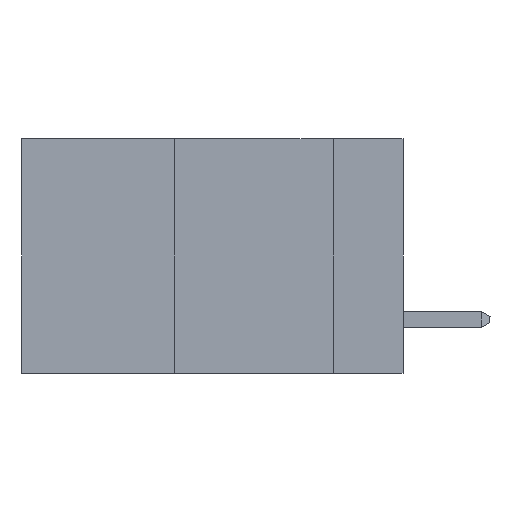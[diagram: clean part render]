
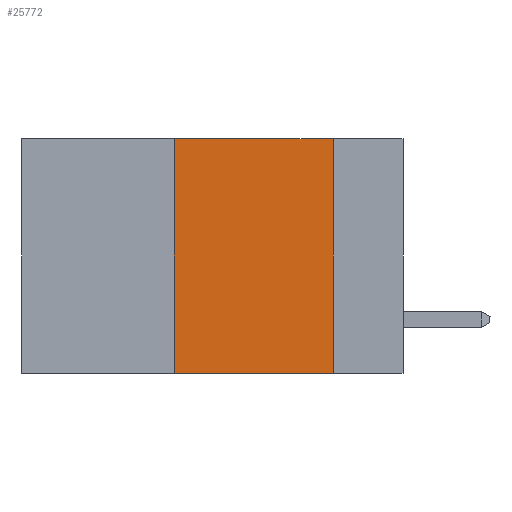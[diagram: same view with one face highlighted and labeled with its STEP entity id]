
A CAD part, left-side view. The second image highlights one B-rep face of the part: STEP entity #25772.
In plain terms, the highlighted planar face has unit normal (-1, 0, 0).
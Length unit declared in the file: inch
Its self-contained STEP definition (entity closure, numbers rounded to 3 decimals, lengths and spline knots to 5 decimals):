
#14 = VECTOR ( 'NONE', #22375, 39.37008 ) ;
#524 = EDGE_LOOP ( 'NONE', ( #15929, #22071, #20313, #9872 ) ) ;
#2654 = DIRECTION ( 'NONE',  ( 0., 0., 1. ) ) ;
#3019 = EDGE_CURVE ( 'NONE', #25509, #14269, #8881, .T. ) ;
#3433 = LINE ( 'NONE', #7960, #14 ) ;
#7960 = CARTESIAN_POINT ( 'NONE',  ( 0., 0.6, 0. ) ) ;
#8402 = CARTESIAN_POINT ( 'NONE',  ( 0., 0.11, 0. ) ) ;
#8881 = LINE ( 'NONE', #13435, #9071 ) ;
#9071 = VECTOR ( 'NONE', #18266, 39.37008 ) ;
#9872 = ORIENTED_EDGE ( 'NONE', *, *, #3019, .T. ) ;
#10600 = CARTESIAN_POINT ( 'NONE',  ( 0., 0.11, 0. ) ) ;
#10876 = CARTESIAN_POINT ( 'NONE',  ( 0., 0.11, -0.37 ) ) ;
#12364 = CARTESIAN_POINT ( 'NONE',  ( 0., 0.36, -0.37 ) ) ;
#13435 = CARTESIAN_POINT ( 'NONE',  ( 0., 0.6, -0.37 ) ) ;
#13705 = VERTEX_POINT ( 'NONE', #10600 ) ;
#13859 = AXIS2_PLACEMENT_3D ( 'NONE', #21410, #26269, #28163 ) ;
#14269 = VERTEX_POINT ( 'NONE', #10876 ) ;
#14543 = CARTESIAN_POINT ( 'NONE',  ( 0., 0.36, 0. ) ) ;
#15761 = LINE ( 'NONE', #8402, #27824 ) ;
#15929 = ORIENTED_EDGE ( 'NONE', *, *, #23107, .F. ) ;
#16095 = FACE_OUTER_BOUND ( 'NONE', #524, .T. ) ;
#16641 = VECTOR ( 'NONE', #2654, 39.37008 ) ;
#18266 = DIRECTION ( 'NONE',  ( 0., -1., 0. ) ) ;
#20121 = EDGE_CURVE ( 'NONE', #25509, #27341, #28943, .T. ) ;
#20313 = ORIENTED_EDGE ( 'NONE', *, *, #20121, .F. ) ;
#21410 = CARTESIAN_POINT ( 'NONE',  ( 0., 0.6, 0. ) ) ;
#22071 = ORIENTED_EDGE ( 'NONE', *, *, #29414, .F. ) ;
#22375 = DIRECTION ( 'NONE',  ( 0., -1., 0. ) ) ;
#22495 = DIRECTION ( 'NONE',  ( 0., 0., -1. ) ) ;
#23107 = EDGE_CURVE ( 'NONE', #13705, #14269, #15761, .T. ) ;
#25509 = VERTEX_POINT ( 'NONE', #12364 ) ;
#25772 = ADVANCED_FACE ( 'NONE', ( #16095 ), #30819, .F. ) ;
#26269 = DIRECTION ( 'NONE',  ( 1., 0., 0. ) ) ;
#27341 = VERTEX_POINT ( 'NONE', #27680 ) ;
#27680 = CARTESIAN_POINT ( 'NONE',  ( 0., 0.36, 0. ) ) ;
#27824 = VECTOR ( 'NONE', #22495, 39.37008 ) ;
#28163 = DIRECTION ( 'NONE',  ( 0., 0., -1. ) ) ;
#28943 = LINE ( 'NONE', #14543, #16641 ) ;
#29414 = EDGE_CURVE ( 'NONE', #27341, #13705, #3433, .T. ) ;
#30819 = PLANE ( 'NONE',  #13859 ) ;
